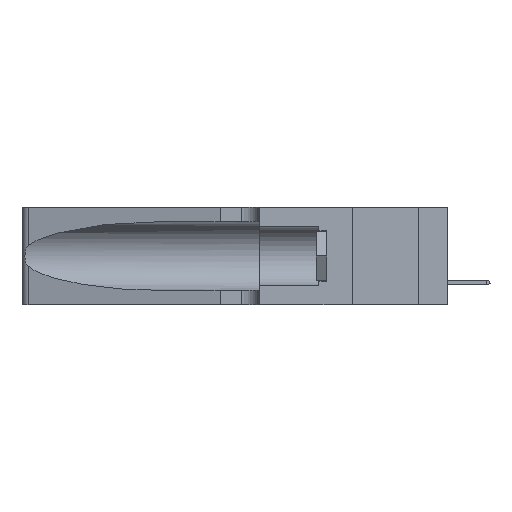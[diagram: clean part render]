
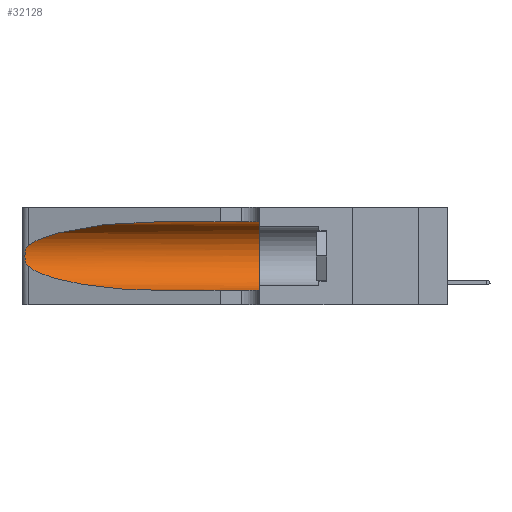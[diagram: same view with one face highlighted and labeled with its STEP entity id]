
A CAD part, left-side view. The second image highlights one B-rep face of the part: STEP entity #32128.
In plain terms, the highlighted cylindrical face has radius 3.308 mm (diameter 6.617 mm), a partial arc.
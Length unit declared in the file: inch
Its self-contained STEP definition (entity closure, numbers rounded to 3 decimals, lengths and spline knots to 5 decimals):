
#424 = VECTOR ( 'NONE', #5575, 39.37008 ) ;
#1856 = CARTESIAN_POINT ( 'NONE',  ( 0.18966, 0.96281, 0.31525 ) ) ;
#3875 = CARTESIAN_POINT ( 'NONE',  ( 0.25555, 1.22993, 0.14849 ) ) ;
#4130 = CARTESIAN_POINT ( 'NONE',  ( 0.25487, 1.22718, 0.22369 ) ) ;
#4147 = CARTESIAN_POINT ( 'NONE',  ( 0.25487, 1.22718, 0.14631 ) ) ;
#5250 = ORIENTED_EDGE ( 'NONE', *, *, #20057, .T. ) ;
#5575 = DIRECTION ( 'NONE',  ( 0., -1., 0. ) ) ;
#6814 = DIRECTION ( 'NONE',  ( 0., 1., 0. ) ) ;
#6839 = ORIENTED_EDGE ( 'NONE', *, *, #21549, .F. ) ;
#6928 = LINE ( 'NONE', #15060, #21272 ) ;
#7074 = DIRECTION ( 'NONE',  ( 0., 0., 1. ) ) ;
#7105 = CARTESIAN_POINT ( 'NONE',  ( 0.26075, 1.23896, 0.19203 ) ) ;
#7973 =( BOUNDED_CURVE ( )  B_SPLINE_CURVE ( 3, ( #17508, #24323, #14205, #24466 ),
 .UNSPECIFIED., .F., .F. ) 
 B_SPLINE_CURVE_WITH_KNOTS ( ( 4, 4 ),
 ( 3.44316, 4.71239 ),
 .UNSPECIFIED. ) 
 CURVE ( )  GEOMETRIC_REPRESENTATION_ITEM ( )  RATIONAL_B_SPLINE_CURVE ( ( 1., 0.87, 0.87, 1. ) ) 
 REPRESENTATION_ITEM ( '' )  );
#8783 = CARTESIAN_POINT ( 'NONE',  ( 0.25487, 1.22718, 0.22369 ) ) ;
#9521 = CARTESIAN_POINT ( 'NONE',  ( 0.25639, 1.23184, 0.21858 ) ) ;
#9598 = DIRECTION ( 'NONE',  ( 0., 0., -1. ) ) ;
#9602 = AXIS2_PLACEMENT_3D ( 'NONE', #13434, #30065, #9598 ) ;
#10784 = CARTESIAN_POINT ( 'NONE',  ( 0.25856, 1.23593, 0.16098 ) ) ;
#10914 = VERTEX_POINT ( 'NONE', #31608 ) ;
#12233 = EDGE_CURVE ( 'NONE', #18487, #10914, #23773, .T. ) ;
#13131 = LINE ( 'NONE', #39343, #424 ) ;
#13434 = CARTESIAN_POINT ( 'NONE',  ( 0.1305, 1.61858, 0.185 ) ) ;
#13802 = CARTESIAN_POINT ( 'NONE',  ( 0.1305, 0.72297, 0.31525 ) ) ;
#14205 = CARTESIAN_POINT ( 'NONE',  ( 0.18966, 0.96281, 0.05475 ) ) ;
#14693 = CARTESIAN_POINT ( 'NONE',  ( 0.1305, 0.35, 0.05475 ) ) ;
#15060 = CARTESIAN_POINT ( 'NONE',  ( 0.1305, 1.61858, 0.05475 ) ) ;
#15558 = CARTESIAN_POINT ( 'NONE',  ( 0.1305, 0.35, 0.31525 ) ) ;
#15924 =( BOUNDED_CURVE ( )  B_SPLINE_CURVE ( 3, ( #29090, #1856, #27014, #4130 ),
 .UNSPECIFIED., .F., .F. ) 
 B_SPLINE_CURVE_WITH_KNOTS ( ( 4, 4 ),
 ( 1.5708, 2.84003 ),
 .UNSPECIFIED. ) 
 CURVE ( )  GEOMETRIC_REPRESENTATION_ITEM ( )  RATIONAL_B_SPLINE_CURVE ( ( 1., 0.87, 0.87, 1. ) ) 
 REPRESENTATION_ITEM ( '' )  );
#16955 = CARTESIAN_POINT ( 'NONE',  ( 0.26018, 1.23835, 0.19895 ) ) ;
#17391 = FACE_OUTER_BOUND ( 'NONE', #20405, .T. ) ;
#17508 = CARTESIAN_POINT ( 'NONE',  ( 0.25487, 1.22718, 0.14631 ) ) ;
#17762 = VERTEX_POINT ( 'NONE', #32497 ) ;
#18353 = DIRECTION ( 'NONE',  ( 0., -1., 0. ) ) ;
#18487 = VERTEX_POINT ( 'NONE', #36160 ) ;
#20057 = EDGE_CURVE ( 'NONE', #21889, #18487, #15924, .T. ) ;
#20405 = EDGE_LOOP ( 'NONE', ( #5250, #31016, #39183, #42172, #33701, #6839 ) ) ;
#20762 = CARTESIAN_POINT ( 'NONE',  ( 0.26075, 1.23896, 0.178 ) ) ;
#21272 = VECTOR ( 'NONE', #18353, 39.37008 ) ;
#21549 = EDGE_CURVE ( 'NONE', #21889, #34777, #13131, .T. ) ;
#21695 = EDGE_CURVE ( 'NONE', #34777, #36131, #33323, .T. ) ;
#21889 = VERTEX_POINT ( 'NONE', #13802 ) ;
#22775 = CARTESIAN_POINT ( 'NONE',  ( 0.25854, 1.2359, 0.20912 ) ) ;
#23734 = CARTESIAN_POINT ( 'NONE',  ( 0.1305, 0.35, 0.185 ) ) ;
#23773 = B_SPLINE_CURVE_WITH_KNOTS ( 'NONE', 3,
 ( #8783, #25416, #9521, #40037, #22775, #16955, #7105, #20762, #30821, #10784, #23884, #41313, #3875, #4147 ),
 .UNSPECIFIED., .F., .F.,
 ( 4, 2, 2, 2, 2, 2, 4 ),
 ( 0., 0.00027, 0.00053, 0.00107, 0.0016, 0.00187, 0.00214 ),
 .UNSPECIFIED. ) ;
#23884 = CARTESIAN_POINT ( 'NONE',  ( 0.25789, 1.23486, 0.15765 ) ) ;
#24323 = CARTESIAN_POINT ( 'NONE',  ( 0.2373, 1.15595, 0.08982 ) ) ;
#24466 = CARTESIAN_POINT ( 'NONE',  ( 0.1305, 0.72297, 0.05475 ) ) ;
#25416 = CARTESIAN_POINT ( 'NONE',  ( 0.25555, 1.22994, 0.2215 ) ) ;
#27014 = CARTESIAN_POINT ( 'NONE',  ( 0.2373, 1.15595, 0.28018 ) ) ;
#29090 = CARTESIAN_POINT ( 'NONE',  ( 0.1305, 0.72297, 0.31525 ) ) ;
#30065 = DIRECTION ( 'NONE',  ( 0., -1., 0. ) ) ;
#30545 = EDGE_CURVE ( 'NONE', #17762, #36131, #6928, .T. ) ;
#30821 = CARTESIAN_POINT ( 'NONE',  ( 0.26017, 1.23833, 0.17102 ) ) ;
#30966 = AXIS2_PLACEMENT_3D ( 'NONE', #23734, #6814, #7074 ) ;
#31016 = ORIENTED_EDGE ( 'NONE', *, *, #12233, .T. ) ;
#31608 = CARTESIAN_POINT ( 'NONE',  ( 0.25487, 1.22718, 0.14631 ) ) ;
#32128 = ADVANCED_FACE ( 'NONE', ( #17391 ), #33811, .F. ) ;
#32497 = CARTESIAN_POINT ( 'NONE',  ( 0.1305, 0.72297, 0.05475 ) ) ;
#33323 = CIRCLE ( 'NONE', #30966, 0.13025 ) ;
#33701 = ORIENTED_EDGE ( 'NONE', *, *, #21695, .F. ) ;
#33811 = CYLINDRICAL_SURFACE ( 'NONE', #9602, 0.13025 ) ;
#34777 = VERTEX_POINT ( 'NONE', #15558 ) ;
#36131 = VERTEX_POINT ( 'NONE', #14693 ) ;
#36160 = CARTESIAN_POINT ( 'NONE',  ( 0.25487, 1.22718, 0.22369 ) ) ;
#36916 = EDGE_CURVE ( 'NONE', #10914, #17762, #7973, .T. ) ;
#39183 = ORIENTED_EDGE ( 'NONE', *, *, #36916, .T. ) ;
#39343 = CARTESIAN_POINT ( 'NONE',  ( 0.1305, 1.61858, 0.31525 ) ) ;
#40037 = CARTESIAN_POINT ( 'NONE',  ( 0.25787, 1.23484, 0.2124 ) ) ;
#41313 = CARTESIAN_POINT ( 'NONE',  ( 0.25639, 1.23186, 0.15144 ) ) ;
#42172 = ORIENTED_EDGE ( 'NONE', *, *, #30545, .T. ) ;
